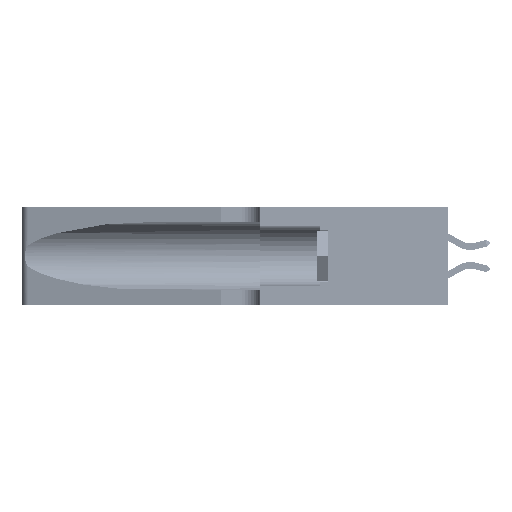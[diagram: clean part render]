
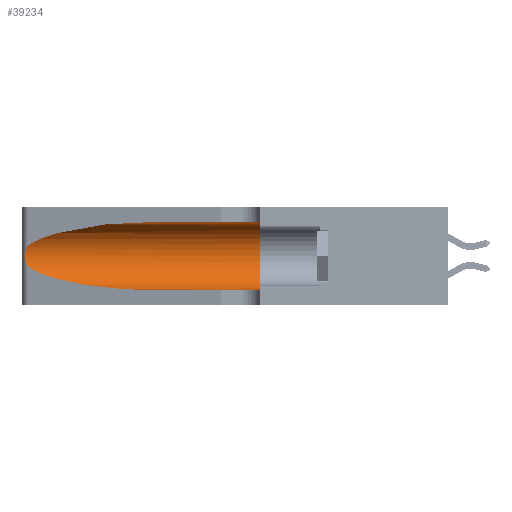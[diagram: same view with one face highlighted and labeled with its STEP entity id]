
A CAD part, left-side view. The second image highlights one B-rep face of the part: STEP entity #39234.
In plain terms, the highlighted cylindrical face has radius 3.308 mm (diameter 6.617 mm), a partial arc.
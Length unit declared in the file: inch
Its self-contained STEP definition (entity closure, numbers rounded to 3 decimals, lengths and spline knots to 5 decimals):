
#640 = CARTESIAN_POINT ( 'NONE',  ( 0.1305, 0.72297, 0.31525 ) ) ;
#854 = DIRECTION ( 'NONE',  ( 0., 0., 1. ) ) ;
#3791 = DIRECTION ( 'NONE',  ( 0., -1., 0. ) ) ;
#4298 = EDGE_CURVE ( 'NONE', #45582, #30089, #20844, .T. ) ;
#4303 = CARTESIAN_POINT ( 'NONE',  ( 0.2373, 1.15595, 0.28018 ) ) ;
#4967 = AXIS2_PLACEMENT_3D ( 'NONE', #15215, #44638, #854 ) ;
#6184 = CARTESIAN_POINT ( 'NONE',  ( 0.25487, 1.22718, 0.14631 ) ) ;
#7235 = DIRECTION ( 'NONE',  ( 0., -1., 0. ) ) ;
#8943 = CARTESIAN_POINT ( 'NONE',  ( 0.25639, 1.23186, 0.15144 ) ) ;
#11045 = CARTESIAN_POINT ( 'NONE',  ( 0.1305, 1.61858, 0.31525 ) ) ;
#11175 = CARTESIAN_POINT ( 'NONE',  ( 0.18966, 0.96281, 0.31525 ) ) ;
#11762 = VECTOR ( 'NONE', #43990, 39.37008 ) ;
#12481 = CARTESIAN_POINT ( 'NONE',  ( 0.25787, 1.23484, 0.2124 ) ) ;
#12662 = CARTESIAN_POINT ( 'NONE',  ( 0.1305, 0.72297, 0.05475 ) ) ;
#12749 = ORIENTED_EDGE ( 'NONE', *, *, #39261, .F. ) ;
#12813 = VERTEX_POINT ( 'NONE', #13324 ) ;
#13227 = ORIENTED_EDGE ( 'NONE', *, *, #34846, .F. ) ;
#13324 = CARTESIAN_POINT ( 'NONE',  ( 0.1305, 0.35, 0.05475 ) ) ;
#13484 = VECTOR ( 'NONE', #3791, 39.37008 ) ;
#14412 = CARTESIAN_POINT ( 'NONE',  ( 0.1305, 1.61858, 0.185 ) ) ;
#14483 = CARTESIAN_POINT ( 'NONE',  ( 0.1305, 0.35, 0.31525 ) ) ;
#15215 = CARTESIAN_POINT ( 'NONE',  ( 0.1305, 0.35, 0.185 ) ) ;
#15745 = EDGE_CURVE ( 'NONE', #42592, #43938, #29422, .T. ) ;
#15771 = LINE ( 'NONE', #18459, #13484 ) ;
#15999 = CARTESIAN_POINT ( 'NONE',  ( 0.25555, 1.22994, 0.2215 ) ) ;
#16073 = AXIS2_PLACEMENT_3D ( 'NONE', #14412, #7235, #43530 ) ;
#16150 = CARTESIAN_POINT ( 'NONE',  ( 0.25856, 1.23593, 0.16098 ) ) ;
#16470 = CARTESIAN_POINT ( 'NONE',  ( 0.26018, 1.23835, 0.19895 ) ) ;
#16579 = EDGE_LOOP ( 'NONE', ( #21933, #33115, #22882, #40447, #13227, #12749 ) ) ;
#17202 = CARTESIAN_POINT ( 'NONE',  ( 0.2373, 1.15595, 0.08982 ) ) ;
#18459 = CARTESIAN_POINT ( 'NONE',  ( 0.1305, 1.61858, 0.05475 ) ) ;
#18631 = CYLINDRICAL_SURFACE ( 'NONE', #16073, 0.13025 ) ;
#20212 = CARTESIAN_POINT ( 'NONE',  ( 0.1305, 0.72297, 0.05475 ) ) ;
#20844 =( BOUNDED_CURVE ( )  B_SPLINE_CURVE ( 3, ( #640, #11175, #4303, #25997 ),
 .UNSPECIFIED., .F., .T. ) 
 B_SPLINE_CURVE_WITH_KNOTS ( ( 4, 4 ),
 ( 1.5708, 2.84003 ),
 .UNSPECIFIED. ) 
 CURVE ( )  GEOMETRIC_REPRESENTATION_ITEM ( )  RATIONAL_B_SPLINE_CURVE ( ( 1., 0.87, 0.87, 1. ) ) 
 REPRESENTATION_ITEM ( '' )  );
#21463 = LINE ( 'NONE', #11045, #11762 ) ;
#21791 = CARTESIAN_POINT ( 'NONE',  ( 0.25487, 1.22718, 0.22369 ) ) ;
#21933 = ORIENTED_EDGE ( 'NONE', *, *, #4298, .T. ) ;
#22092 = EDGE_CURVE ( 'NONE', #30089, #42592, #23566, .T. ) ;
#22882 = ORIENTED_EDGE ( 'NONE', *, *, #15745, .T. ) ;
#23318 = CARTESIAN_POINT ( 'NONE',  ( 0.25854, 1.2359, 0.20912 ) ) ;
#23476 = CARTESIAN_POINT ( 'NONE',  ( 0.26075, 1.23896, 0.178 ) ) ;
#23566 = B_SPLINE_CURVE_WITH_KNOTS ( 'NONE', 3,
 ( #44952, #15999, #27296, #12481, #23318, #16470, #41449, #23476, #44798, #16150, #27146, #8943, #30954, #45424 ),
 .UNSPECIFIED., .F., .F.,
 ( 4, 2, 2, 2, 2, 2, 4 ),
 ( 0., 0.00027, 0.00053, 0.00107, 0.0016, 0.00187, 0.00214 ),
 .UNSPECIFIED. ) ;
#25997 = CARTESIAN_POINT ( 'NONE',  ( 0.25487, 1.22718, 0.22369 ) ) ;
#27146 = CARTESIAN_POINT ( 'NONE',  ( 0.25789, 1.23486, 0.15765 ) ) ;
#27296 = CARTESIAN_POINT ( 'NONE',  ( 0.25639, 1.23184, 0.21858 ) ) ;
#29422 =( BOUNDED_CURVE ( )  B_SPLINE_CURVE ( 3, ( #6184, #17202, #35485, #20212 ),
 .UNSPECIFIED., .F., .F. ) 
 B_SPLINE_CURVE_WITH_KNOTS ( ( 4, 4 ),
 ( 3.44316, 4.71239 ),
 .UNSPECIFIED. ) 
 CURVE ( )  GEOMETRIC_REPRESENTATION_ITEM ( )  RATIONAL_B_SPLINE_CURVE ( ( 1., 0.87, 0.87, 1. ) ) 
 REPRESENTATION_ITEM ( '' )  );
#30083 = VERTEX_POINT ( 'NONE', #14483 ) ;
#30089 = VERTEX_POINT ( 'NONE', #21791 ) ;
#30954 = CARTESIAN_POINT ( 'NONE',  ( 0.25555, 1.22993, 0.14849 ) ) ;
#33115 = ORIENTED_EDGE ( 'NONE', *, *, #22092, .T. ) ;
#34846 = EDGE_CURVE ( 'NONE', #30083, #12813, #42105, .T. ) ;
#35485 = CARTESIAN_POINT ( 'NONE',  ( 0.18966, 0.96281, 0.05475 ) ) ;
#36276 = EDGE_CURVE ( 'NONE', #43938, #12813, #15771, .T. ) ;
#37978 = FACE_OUTER_BOUND ( 'NONE', #16579, .T. ) ;
#38575 = CARTESIAN_POINT ( 'NONE',  ( 0.1305, 0.72297, 0.31525 ) ) ;
#39234 = ADVANCED_FACE ( 'NONE', ( #37978 ), #18631, .F. ) ;
#39261 = EDGE_CURVE ( 'NONE', #45582, #30083, #21463, .T. ) ;
#40447 = ORIENTED_EDGE ( 'NONE', *, *, #36276, .T. ) ;
#41449 = CARTESIAN_POINT ( 'NONE',  ( 0.26075, 1.23896, 0.19203 ) ) ;
#42105 = CIRCLE ( 'NONE', #4967, 0.13025 ) ;
#42592 = VERTEX_POINT ( 'NONE', #45221 ) ;
#43530 = DIRECTION ( 'NONE',  ( 0., 0., -1. ) ) ;
#43938 = VERTEX_POINT ( 'NONE', #12662 ) ;
#43990 = DIRECTION ( 'NONE',  ( 0., -1., 0. ) ) ;
#44638 = DIRECTION ( 'NONE',  ( 0., 1., 0. ) ) ;
#44798 = CARTESIAN_POINT ( 'NONE',  ( 0.26017, 1.23833, 0.17102 ) ) ;
#44952 = CARTESIAN_POINT ( 'NONE',  ( 0.25487, 1.22718, 0.22369 ) ) ;
#45221 = CARTESIAN_POINT ( 'NONE',  ( 0.25487, 1.22718, 0.14631 ) ) ;
#45424 = CARTESIAN_POINT ( 'NONE',  ( 0.25487, 1.22718, 0.14631 ) ) ;
#45582 = VERTEX_POINT ( 'NONE', #38575 ) ;
